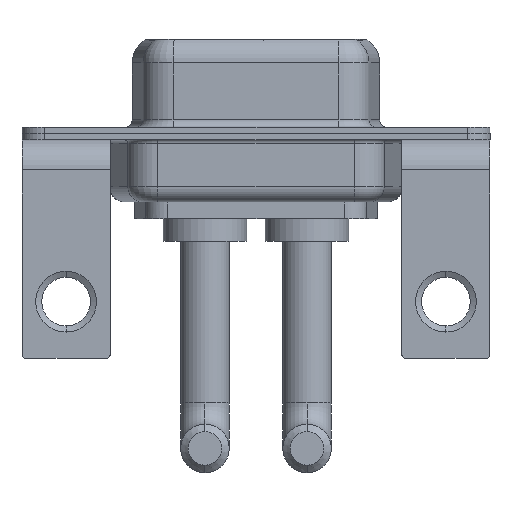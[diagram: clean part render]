
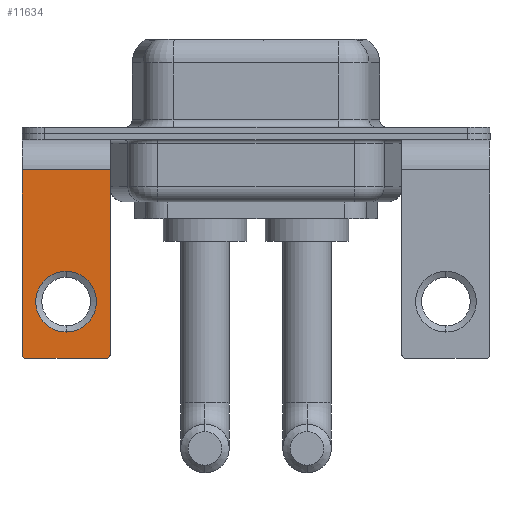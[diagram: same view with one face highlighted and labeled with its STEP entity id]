
A CAD part, front view. The second image highlights one B-rep face of the part: STEP entity #11634.
In plain terms, the highlighted planar face has unit normal (0, -1, 0).
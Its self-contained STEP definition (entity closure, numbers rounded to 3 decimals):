
#24 = VERTEX_POINT ( 'NONE', #12337 ) ;
#140 = EDGE_CURVE ( 'NONE', #24, #2098, #10404, .T. ) ;
#229 = DIRECTION ( 'NONE',  ( 0., 0., 1. ) ) ;
#281 = DIRECTION ( 'NONE',  ( 0., -1., 0. ) ) ;
#308 = CARTESIAN_POINT ( 'NONE',  ( 0., -6.25, -9.07 ) ) ;
#343 = CARTESIAN_POINT ( 'NONE',  ( -2.65, -6.25, -14.55 ) ) ;
#398 = VERTEX_POINT ( 'NONE', #13459 ) ;
#404 = VECTOR ( 'NONE', #12702, 1000. ) ;
#417 = ORIENTED_EDGE ( 'NONE', *, *, #8904, .F. ) ;
#794 = AXIS2_PLACEMENT_3D ( 'NONE', #343, #7875, #5817 ) ;
#802 = VERTEX_POINT ( 'NONE', #4121 ) ;
#944 = DIRECTION ( 'NONE',  ( 0., 0., -1. ) ) ;
#1883 = ORIENTED_EDGE ( 'NONE', *, *, #6693, .T. ) ;
#2019 = VERTEX_POINT ( 'NONE', #308 ) ;
#2020 = CARTESIAN_POINT ( 'NONE',  ( 2.9, -6.25, -2.4 ) ) ;
#2085 = VERTEX_POINT ( 'NONE', #2864 ) ;
#2098 = VERTEX_POINT ( 'NONE', #8062 ) ;
#2634 = VERTEX_POINT ( 'NONE', #2771 ) ;
#2771 = CARTESIAN_POINT ( 'NONE',  ( 2.9, -6.25, -14.55 ) ) ;
#2864 = CARTESIAN_POINT ( 'NONE',  ( -2.65, -6.25, -14.8 ) ) ;
#2947 = ORIENTED_EDGE ( 'NONE', *, *, #11816, .T. ) ;
#2977 = VECTOR ( 'NONE', #7812, 1000. ) ;
#3021 = ORIENTED_EDGE ( 'NONE', *, *, #3781, .T. ) ;
#3277 = AXIS2_PLACEMENT_3D ( 'NONE', #4632, #281, #3497 ) ;
#3361 = DIRECTION ( 'NONE',  ( 0., 1., 0. ) ) ;
#3497 = DIRECTION ( 'NONE',  ( 0., 0., 1. ) ) ;
#3739 = ORIENTED_EDGE ( 'NONE', *, *, #4863, .T. ) ;
#3781 = EDGE_CURVE ( 'NONE', #2019, #802, #6879, .T. ) ;
#3818 = CARTESIAN_POINT ( 'NONE',  ( -2.9, -6.25, -2.4 ) ) ;
#4121 = CARTESIAN_POINT ( 'NONE',  ( 0., -6.25, -13.07 ) ) ;
#4248 = VECTOR ( 'NONE', #944, 1000. ) ;
#4462 = ORIENTED_EDGE ( 'NONE', *, *, #140, .T. ) ;
#4616 = VERTEX_POINT ( 'NONE', #6601 ) ;
#4632 = CARTESIAN_POINT ( 'NONE',  ( 2.65, -6.25, -14.55 ) ) ;
#4809 = DIRECTION ( 'NONE',  ( 0., 0., -1. ) ) ;
#4863 = EDGE_CURVE ( 'NONE', #2098, #398, #13440, .T. ) ;
#4874 = VECTOR ( 'NONE', #4809, 1000. ) ;
#4930 = FACE_OUTER_BOUND ( 'NONE', #5871, .T. ) ;
#5587 = DIRECTION ( 'NONE',  ( 0., 1., 0. ) ) ;
#5636 = CARTESIAN_POINT ( 'NONE',  ( 0., -6.25, -11.07 ) ) ;
#5748 = AXIS2_PLACEMENT_3D ( 'NONE', #12556, #3361, #12053 ) ;
#5817 = DIRECTION ( 'NONE',  ( 0., 0., 1. ) ) ;
#5871 = EDGE_LOOP ( 'NONE', ( #3739, #11286, #417, #2947, #9218, #4462 ) ) ;
#5889 = EDGE_CURVE ( 'NONE', #398, #2085, #10588, .T. ) ;
#6566 = EDGE_CURVE ( 'NONE', #24, #2634, #11730, .T. ) ;
#6601 = CARTESIAN_POINT ( 'NONE',  ( 2.65, -6.25, -14.8 ) ) ;
#6612 = CARTESIAN_POINT ( 'NONE',  ( 2.9, -6.25, -14.8 ) ) ;
#6693 = EDGE_CURVE ( 'NONE', #802, #2019, #13351, .T. ) ;
#6879 = CIRCLE ( 'NONE', #12399, 2. ) ;
#7182 = AXIS2_PLACEMENT_3D ( 'NONE', #12139, #5587, #12220 ) ;
#7183 = CARTESIAN_POINT ( 'NONE',  ( 2.9, -6.25, -2.4 ) ) ;
#7812 = DIRECTION ( 'NONE',  ( -1., 0., 0. ) ) ;
#7875 = DIRECTION ( 'NONE',  ( 0., -1., 0. ) ) ;
#8062 = CARTESIAN_POINT ( 'NONE',  ( -2.9, -6.25, -2.4 ) ) ;
#8904 = EDGE_CURVE ( 'NONE', #4616, #2085, #12906, .T. ) ;
#9218 = ORIENTED_EDGE ( 'NONE', *, *, #6566, .F. ) ;
#9549 = FACE_BOUND ( 'NONE', #12340, .T. ) ;
#9978 = DIRECTION ( 'NONE',  ( 0., 1., 0. ) ) ;
#10404 = LINE ( 'NONE', #7183, #404 ) ;
#10588 = CIRCLE ( 'NONE', #794, 0.25 ) ;
#11286 = ORIENTED_EDGE ( 'NONE', *, *, #5889, .T. ) ;
#11634 = ADVANCED_FACE ( 'NONE', ( #9549, #4930 ), #13629, .F. ) ;
#11730 = LINE ( 'NONE', #2020, #4248 ) ;
#11816 = EDGE_CURVE ( 'NONE', #4616, #2634, #13961, .T. ) ;
#12053 = DIRECTION ( 'NONE',  ( 0., 0., 1. ) ) ;
#12139 = CARTESIAN_POINT ( 'NONE',  ( 0., -6.25, -11.07 ) ) ;
#12220 = DIRECTION ( 'NONE',  ( 0., 0., 1. ) ) ;
#12337 = CARTESIAN_POINT ( 'NONE',  ( 2.9, -6.25, -2.4 ) ) ;
#12340 = EDGE_LOOP ( 'NONE', ( #1883, #3021 ) ) ;
#12399 = AXIS2_PLACEMENT_3D ( 'NONE', #5636, #9978, #229 ) ;
#12556 = CARTESIAN_POINT ( 'NONE',  ( 2.9, -6.25, -2.4 ) ) ;
#12702 = DIRECTION ( 'NONE',  ( -1., 0., 0. ) ) ;
#12906 = LINE ( 'NONE', #6612, #2977 ) ;
#13351 = CIRCLE ( 'NONE', #7182, 2. ) ;
#13440 = LINE ( 'NONE', #3818, #4874 ) ;
#13459 = CARTESIAN_POINT ( 'NONE',  ( -2.9, -6.25, -14.55 ) ) ;
#13629 = PLANE ( 'NONE',  #5748 ) ;
#13961 = CIRCLE ( 'NONE', #3277, 0.25 ) ;
